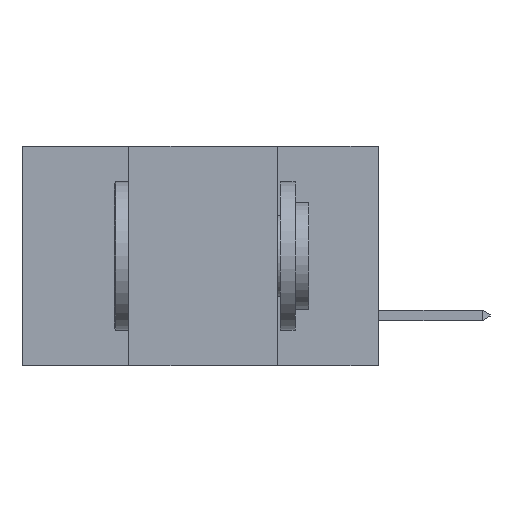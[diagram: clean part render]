
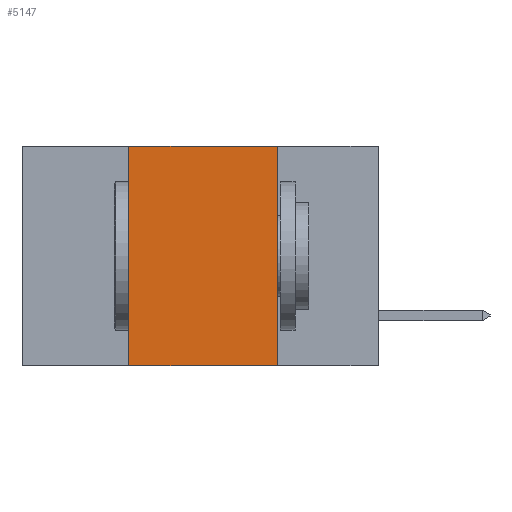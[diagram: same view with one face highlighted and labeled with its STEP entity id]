
A CAD part, left-side view. The second image highlights one B-rep face of the part: STEP entity #5147.
In plain terms, the highlighted planar face has unit normal (-1, 0, 0).
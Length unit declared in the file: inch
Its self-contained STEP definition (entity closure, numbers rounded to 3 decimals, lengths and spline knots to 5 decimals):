
#102 = EDGE_CURVE ( 'NONE', #8654, #1739, #13689, .T. ) ;
#218 = ORIENTED_EDGE ( 'NONE', *, *, #102, .T. ) ;
#387 = EDGE_LOOP ( 'NONE', ( #11570, #15551, #16021, #218 ) ) ;
#992 = CARTESIAN_POINT ( 'NONE',  ( 0., 0.42, -0.37 ) ) ;
#1739 = VERTEX_POINT ( 'NONE', #18753 ) ;
#1813 = FACE_OUTER_BOUND ( 'NONE', #387, .T. ) ;
#1952 = DIRECTION ( 'NONE',  ( 0., -1., 0. ) ) ;
#3072 = VERTEX_POINT ( 'NONE', #16369 ) ;
#3140 = CARTESIAN_POINT ( 'NONE',  ( 0., 0.17, 0. ) ) ;
#4851 = LINE ( 'NONE', #18310, #8406 ) ;
#5147 = ADVANCED_FACE ( 'NONE', ( #1813 ), #8629, .F. ) ;
#5575 = CARTESIAN_POINT ( 'NONE',  ( 0., 0.6, -0.37 ) ) ;
#5999 = CARTESIAN_POINT ( 'NONE',  ( 0., 0.42, -0.37 ) ) ;
#6764 = LINE ( 'NONE', #992, #10871 ) ;
#7313 = DIRECTION ( 'NONE',  ( 0., -1., 0. ) ) ;
#7492 = CARTESIAN_POINT ( 'NONE',  ( 0., 0.6, 0. ) ) ;
#8033 = EDGE_CURVE ( 'NONE', #11783, #1739, #4851, .T. ) ;
#8406 = VECTOR ( 'NONE', #19812, 39.37008 ) ;
#8503 = DIRECTION ( 'NONE',  ( 0., 0., -1. ) ) ;
#8547 = DIRECTION ( 'NONE',  ( 1., 0., 0. ) ) ;
#8629 = PLANE ( 'NONE',  #13151 ) ;
#8654 = VERTEX_POINT ( 'NONE', #5999 ) ;
#9170 = VECTOR ( 'NONE', #1952, 39.37008 ) ;
#10209 = DIRECTION ( 'NONE',  ( 0., 0., 1. ) ) ;
#10871 = VECTOR ( 'NONE', #10209, 39.37008 ) ;
#11570 = ORIENTED_EDGE ( 'NONE', *, *, #8033, .F. ) ;
#11783 = VERTEX_POINT ( 'NONE', #3140 ) ;
#11821 = EDGE_CURVE ( 'NONE', #8654, #3072, #6764, .T. ) ;
#11946 = CARTESIAN_POINT ( 'NONE',  ( 0., 0.6, 0. ) ) ;
#13151 = AXIS2_PLACEMENT_3D ( 'NONE', #7492, #8547, #8503 ) ;
#13689 = LINE ( 'NONE', #5575, #9170 ) ;
#13791 = EDGE_CURVE ( 'NONE', #3072, #11783, #14547, .T. ) ;
#14547 = LINE ( 'NONE', #11946, #17693 ) ;
#15551 = ORIENTED_EDGE ( 'NONE', *, *, #13791, .F. ) ;
#16021 = ORIENTED_EDGE ( 'NONE', *, *, #11821, .F. ) ;
#16369 = CARTESIAN_POINT ( 'NONE',  ( 0., 0.42, 0. ) ) ;
#17693 = VECTOR ( 'NONE', #7313, 39.37008 ) ;
#18310 = CARTESIAN_POINT ( 'NONE',  ( 0., 0.17, -0.37 ) ) ;
#18753 = CARTESIAN_POINT ( 'NONE',  ( 0., 0.17, -0.37 ) ) ;
#19812 = DIRECTION ( 'NONE',  ( 0., 0., -1. ) ) ;
